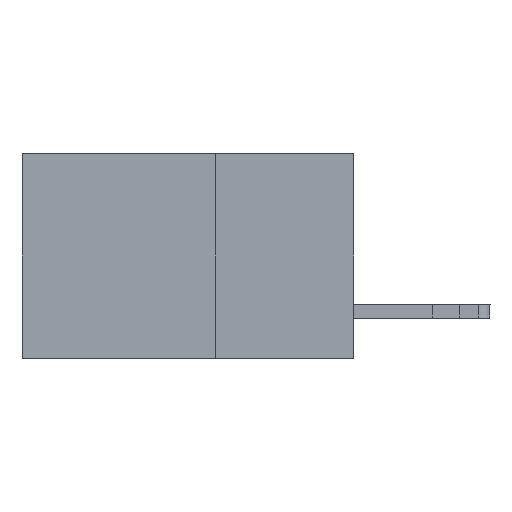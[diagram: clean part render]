
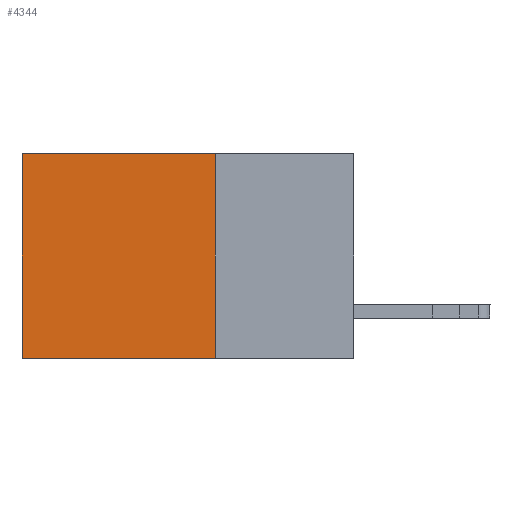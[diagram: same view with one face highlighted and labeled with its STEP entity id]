
A CAD part, left-side view. The second image highlights one B-rep face of the part: STEP entity #4344.
In plain terms, the highlighted planar face has unit normal (-1, 0, 0).
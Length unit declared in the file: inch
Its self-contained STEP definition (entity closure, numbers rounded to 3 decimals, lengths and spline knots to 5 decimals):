
#57 = FACE_OUTER_BOUND ( 'NONE', #12310, .T. ) ;
#109 = EDGE_CURVE ( 'NONE', #3261, #10793, #7525, .T. ) ;
#327 = DIRECTION ( 'NONE',  ( 0., 1., 0. ) ) ;
#1037 = CARTESIAN_POINT ( 'NONE',  ( 0.2875, 0.6, -0.37 ) ) ;
#2574 = EDGE_CURVE ( 'NONE', #10793, #3911, #11217, .T. ) ;
#3261 = VERTEX_POINT ( 'NONE', #11371 ) ;
#3911 = VERTEX_POINT ( 'NONE', #1037 ) ;
#3947 = AXIS2_PLACEMENT_3D ( 'NONE', #12049, #14363, #8612 ) ;
#4070 = CARTESIAN_POINT ( 'NONE',  ( 0.2875, 0.25, 0. ) ) ;
#4344 = ADVANCED_FACE ( 'NONE', ( #57 ), #8719, .F. ) ;
#5183 = CARTESIAN_POINT ( 'NONE',  ( 0.2875, 0.6, 0. ) ) ;
#5642 = VECTOR ( 'NONE', #13793, 39.37008 ) ;
#5740 = ORIENTED_EDGE ( 'NONE', *, *, #2574, .T. ) ;
#6362 = LINE ( 'NONE', #9393, #5642 ) ;
#6428 = CARTESIAN_POINT ( 'NONE',  ( 0.2875, 0.25, -0.37 ) ) ;
#6451 = VECTOR ( 'NONE', #8727, 39.37008 ) ;
#7525 = LINE ( 'NONE', #4070, #6451 ) ;
#8308 = VECTOR ( 'NONE', #327, 39.37008 ) ;
#8567 = EDGE_CURVE ( 'NONE', #13089, #3911, #10888, .T. ) ;
#8612 = DIRECTION ( 'NONE',  ( 0., 0., -1. ) ) ;
#8719 = PLANE ( 'NONE',  #3947 ) ;
#8727 = DIRECTION ( 'NONE',  ( 0., 1., 0. ) ) ;
#9393 = CARTESIAN_POINT ( 'NONE',  ( 0.2875, 0.25, 0. ) ) ;
#10691 = EDGE_CURVE ( 'NONE', #3261, #13089, #6362, .T. ) ;
#10793 = VERTEX_POINT ( 'NONE', #5183 ) ;
#10888 = LINE ( 'NONE', #14097, #8308 ) ;
#11217 = LINE ( 'NONE', #13820, #12813 ) ;
#11371 = CARTESIAN_POINT ( 'NONE',  ( 0.2875, 0.25, 0. ) ) ;
#11616 = DIRECTION ( 'NONE',  ( 0., 0., -1. ) ) ;
#12049 = CARTESIAN_POINT ( 'NONE',  ( 0.2875, 0.25, 0. ) ) ;
#12310 = EDGE_LOOP ( 'NONE', ( #5740, #13503, #13246, #13151 ) ) ;
#12813 = VECTOR ( 'NONE', #11616, 39.37008 ) ;
#13089 = VERTEX_POINT ( 'NONE', #6428 ) ;
#13151 = ORIENTED_EDGE ( 'NONE', *, *, #109, .T. ) ;
#13246 = ORIENTED_EDGE ( 'NONE', *, *, #10691, .F. ) ;
#13503 = ORIENTED_EDGE ( 'NONE', *, *, #8567, .F. ) ;
#13793 = DIRECTION ( 'NONE',  ( 0., 0., -1. ) ) ;
#13820 = CARTESIAN_POINT ( 'NONE',  ( 0.2875, 0.6, 0. ) ) ;
#14097 = CARTESIAN_POINT ( 'NONE',  ( 0.2875, 0.25, -0.37 ) ) ;
#14363 = DIRECTION ( 'NONE',  ( 1., 0., 0. ) ) ;
